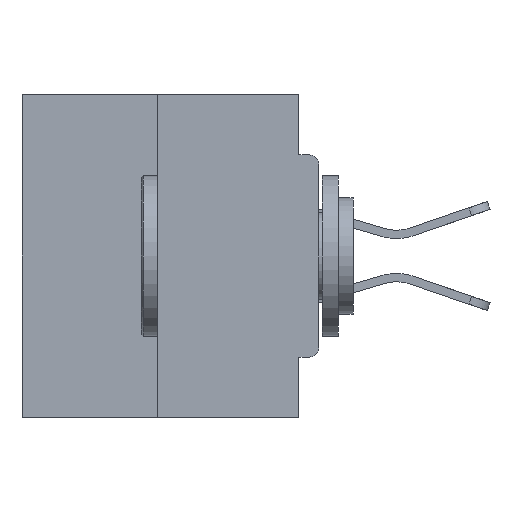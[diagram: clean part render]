
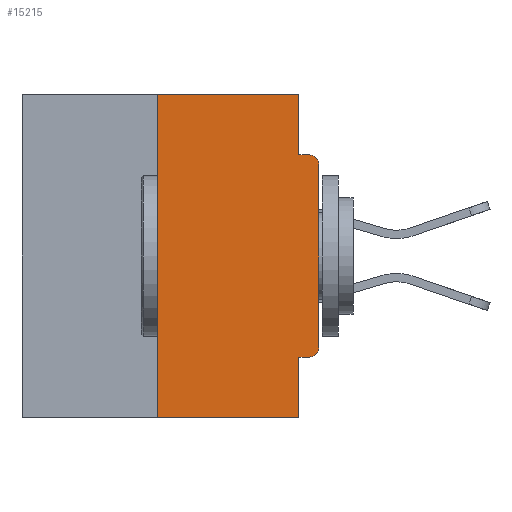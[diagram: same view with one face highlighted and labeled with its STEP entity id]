
A CAD part, left-side view. The second image highlights one B-rep face of the part: STEP entity #15215.
In plain terms, the highlighted planar face has unit normal (-1, 0, 0).
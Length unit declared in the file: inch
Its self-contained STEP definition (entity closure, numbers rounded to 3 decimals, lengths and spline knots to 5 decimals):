
#818 = ORIENTED_EDGE ( 'NONE', *, *, #19219, .F. ) ;
#1291 = CARTESIAN_POINT ( 'NONE',  ( 0., 0.46, 0. ) ) ;
#1396 = PLANE ( 'NONE',  #4076 ) ;
#1493 = CARTESIAN_POINT ( 'NONE',  ( 0., 0.015, -0.0935 ) ) ;
#1761 = LINE ( 'NONE', #28572, #3766 ) ;
#2204 = CARTESIAN_POINT ( 'NONE',  ( 0., 0., 0. ) ) ;
#2978 = ORIENTED_EDGE ( 'NONE', *, *, #10022, .T. ) ;
#3099 = DIRECTION ( 'NONE',  ( 0., -1., 0. ) ) ;
#3766 = VECTOR ( 'NONE', #28338, 39.37008 ) ;
#4076 = AXIS2_PLACEMENT_3D ( 'NONE', #1291, #14390, #6731 ) ;
#4202 = CARTESIAN_POINT ( 'NONE',  ( 0., 0., -0.1085 ) ) ;
#4595 = DIRECTION ( 'NONE',  ( 0., 0., 1. ) ) ;
#5123 = CARTESIAN_POINT ( 'NONE',  ( 0., 0.031, -0.0935 ) ) ;
#5196 = DIRECTION ( 'NONE',  ( 0., -1., 0. ) ) ;
#5231 = DIRECTION ( 'NONE',  ( -1., 0., 0. ) ) ;
#5529 = CARTESIAN_POINT ( 'NONE',  ( 0., 0.031, -0.5 ) ) ;
#6047 = VERTEX_POINT ( 'NONE', #22718 ) ;
#6731 = DIRECTION ( 'NONE',  ( 0., 0., -1. ) ) ;
#6977 = AXIS2_PLACEMENT_3D ( 'NONE', #15515, #28365, #20874 ) ;
#7645 = ORIENTED_EDGE ( 'NONE', *, *, #8172, .F. ) ;
#7917 = VECTOR ( 'NONE', #21572, 39.37008 ) ;
#7987 = CARTESIAN_POINT ( 'NONE',  ( 0., 0.25, 0. ) ) ;
#8164 = ORIENTED_EDGE ( 'NONE', *, *, #31770, .F. ) ;
#8172 = EDGE_CURVE ( 'NONE', #9901, #32308, #22963, .T. ) ;
#8554 = EDGE_CURVE ( 'NONE', #32146, #17877, #19443, .T. ) ;
#8709 = ORIENTED_EDGE ( 'NONE', *, *, #33242, .T. ) ;
#9901 = VERTEX_POINT ( 'NONE', #18437 ) ;
#10022 = EDGE_CURVE ( 'NONE', #9901, #20222, #26228, .T. ) ;
#10581 = CARTESIAN_POINT ( 'NONE',  ( 0., 0.015, -0.4065 ) ) ;
#11263 = ORIENTED_EDGE ( 'NONE', *, *, #23634, .F. ) ;
#12198 = LINE ( 'NONE', #18713, #20374 ) ;
#12552 = EDGE_CURVE ( 'NONE', #16503, #17877, #22643, .T. ) ;
#12789 = LINE ( 'NONE', #24179, #7917 ) ;
#13002 = DIRECTION ( 'NONE',  ( 0., 0., 1. ) ) ;
#13442 = CIRCLE ( 'NONE', #18233, 0.015 ) ;
#13938 = CARTESIAN_POINT ( 'NONE',  ( 0., 0.031, -0.4065 ) ) ;
#14390 = DIRECTION ( 'NONE',  ( 1., 0., 0. ) ) ;
#15215 = ADVANCED_FACE ( 'NONE', ( #30632 ), #1396, .F. ) ;
#15276 = DIRECTION ( 'NONE',  ( 0., 0., -1. ) ) ;
#15515 = CARTESIAN_POINT ( 'NONE',  ( 0., 0.015, -0.1085 ) ) ;
#15944 = CARTESIAN_POINT ( 'NONE',  ( 0., 0.46, -0.5 ) ) ;
#16057 = VECTOR ( 'NONE', #13002, 39.37008 ) ;
#16503 = VERTEX_POINT ( 'NONE', #5123 ) ;
#17081 = ORIENTED_EDGE ( 'NONE', *, *, #32190, .T. ) ;
#17144 = ORIENTED_EDGE ( 'NONE', *, *, #29823, .F. ) ;
#17877 = VERTEX_POINT ( 'NONE', #1493 ) ;
#18233 = AXIS2_PLACEMENT_3D ( 'NONE', #20505, #5231, #15276 ) ;
#18435 = VERTEX_POINT ( 'NONE', #10581 ) ;
#18437 = CARTESIAN_POINT ( 'NONE',  ( 0., 0.25, -0.5 ) ) ;
#18441 = VECTOR ( 'NONE', #18634, 39.37008 ) ;
#18634 = DIRECTION ( 'NONE',  ( 0., 0., -1. ) ) ;
#18713 = CARTESIAN_POINT ( 'NONE',  ( 0., 0.46, 0. ) ) ;
#19219 = EDGE_CURVE ( 'NONE', #6047, #16503, #12789, .T. ) ;
#19443 = CIRCLE ( 'NONE', #6977, 0.015 ) ;
#20222 = VERTEX_POINT ( 'NONE', #26399 ) ;
#20374 = VECTOR ( 'NONE', #3099, 39.37008 ) ;
#20505 = CARTESIAN_POINT ( 'NONE',  ( 0., 0.015, -0.3915 ) ) ;
#20874 = DIRECTION ( 'NONE',  ( 0., 0., -1. ) ) ;
#21474 = ORIENTED_EDGE ( 'NONE', *, *, #12552, .F. ) ;
#21572 = DIRECTION ( 'NONE',  ( 0., 0., -1. ) ) ;
#22541 = VECTOR ( 'NONE', #31973, 39.37008 ) ;
#22643 = LINE ( 'NONE', #28888, #32833 ) ;
#22718 = CARTESIAN_POINT ( 'NONE',  ( 0., 0.031, 0. ) ) ;
#22963 = LINE ( 'NONE', #7987, #16057 ) ;
#23094 = VECTOR ( 'NONE', #4595, 39.37008 ) ;
#23634 = EDGE_CURVE ( 'NONE', #26777, #20222, #28635, .T. ) ;
#24142 = ORIENTED_EDGE ( 'NONE', *, *, #8554, .T. ) ;
#24179 = CARTESIAN_POINT ( 'NONE',  ( 0., 0.031, 0. ) ) ;
#24719 = LINE ( 'NONE', #2204, #23094 ) ;
#25774 = EDGE_LOOP ( 'NONE', ( #8164, #7645, #2978, #11263, #17144, #17081, #8709, #24142, #21474, #818 ) ) ;
#26228 = LINE ( 'NONE', #15944, #22541 ) ;
#26264 = VERTEX_POINT ( 'NONE', #32502 ) ;
#26399 = CARTESIAN_POINT ( 'NONE',  ( 0., 0.031, -0.5 ) ) ;
#26777 = VERTEX_POINT ( 'NONE', #13938 ) ;
#28338 = DIRECTION ( 'NONE',  ( 0., 1., 0. ) ) ;
#28365 = DIRECTION ( 'NONE',  ( -1., 0., 0. ) ) ;
#28572 = CARTESIAN_POINT ( 'NONE',  ( 0., 0., -0.4065 ) ) ;
#28635 = LINE ( 'NONE', #5529, #18441 ) ;
#28816 = CARTESIAN_POINT ( 'NONE',  ( 0., 0.25, 0. ) ) ;
#28888 = CARTESIAN_POINT ( 'NONE',  ( 0., 0., -0.0935 ) ) ;
#29823 = EDGE_CURVE ( 'NONE', #18435, #26777, #1761, .T. ) ;
#30632 = FACE_OUTER_BOUND ( 'NONE', #25774, .T. ) ;
#31770 = EDGE_CURVE ( 'NONE', #32308, #6047, #12198, .T. ) ;
#31973 = DIRECTION ( 'NONE',  ( 0., -1., 0. ) ) ;
#32146 = VERTEX_POINT ( 'NONE', #4202 ) ;
#32190 = EDGE_CURVE ( 'NONE', #18435, #26264, #13442, .T. ) ;
#32308 = VERTEX_POINT ( 'NONE', #28816 ) ;
#32502 = CARTESIAN_POINT ( 'NONE',  ( 0., 0., -0.3915 ) ) ;
#32833 = VECTOR ( 'NONE', #5196, 39.37008 ) ;
#33242 = EDGE_CURVE ( 'NONE', #26264, #32146, #24719, .T. ) ;
